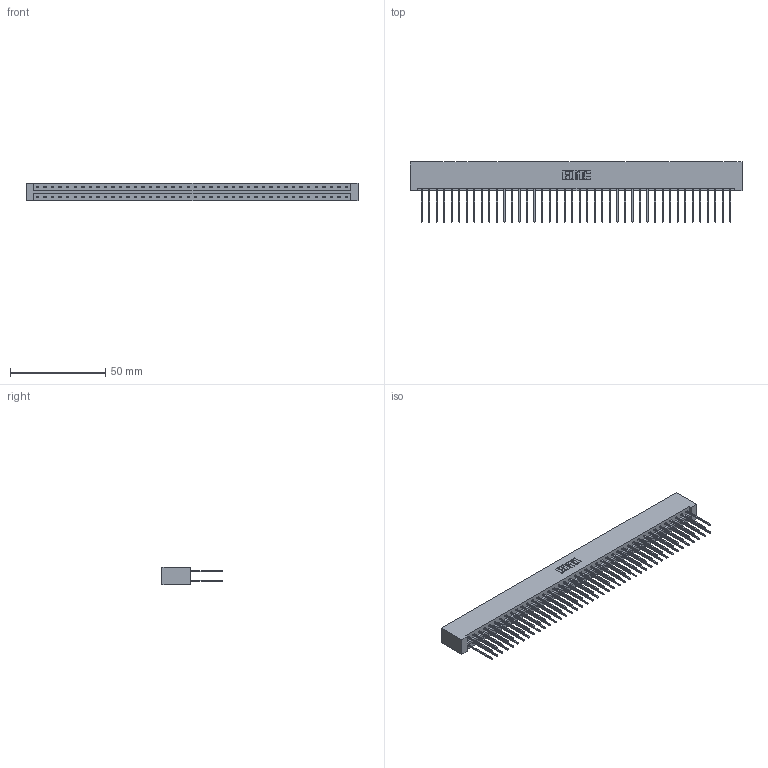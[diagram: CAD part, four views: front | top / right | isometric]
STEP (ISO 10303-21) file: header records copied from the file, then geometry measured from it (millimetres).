
FILE_DESCRIPTION (( 'STEP AP203' ), '1' );
FILE_NAME ('333-084-542-201.STEP', '2018-08-05T04:41:41', ( '' ), ( '' ), 'SwSTEP 2.0', 'SolidWorks 2016', '' );
FILE_SCHEMA (( 'CONFIG_CONTROL_DESIGN' ));
Length unit declared in the file: inch
Products named in the file (3): 333 Part_Lugless; 345-292-001_345-293-142; 333-084-542-201
Assembly tree (85 placements, depth 2):
  333-084-542-201
    333 Part_Lugless
    345-292-001_345-293-142  x84
Bounding box: 174.68 x 31.63 x 9.4 mm (x, y, z)
Volume: 18857.2 mm3; surface area: 24255.7 mm2
Topology: 85 solids, 85 shells, 4474 faces, 13307 edges, 8758 vertices
Faces by surface type: plane 3090, cylinder 1384
Entity records: 26761 total; most frequent: CARTESIAN_POINT 4434, ORIENTED_EDGE 4370, DIRECTION 3781, EDGE_CURVE 2185, VECTOR 2065, LINE 2065, VERTEX_POINT 1454, AXIS2_PLACEMENT_3D 858
